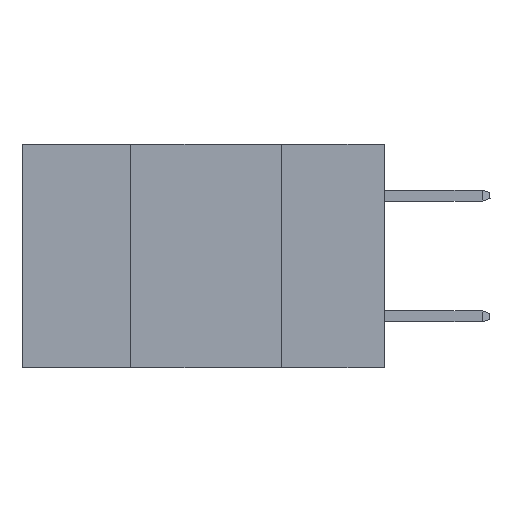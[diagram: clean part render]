
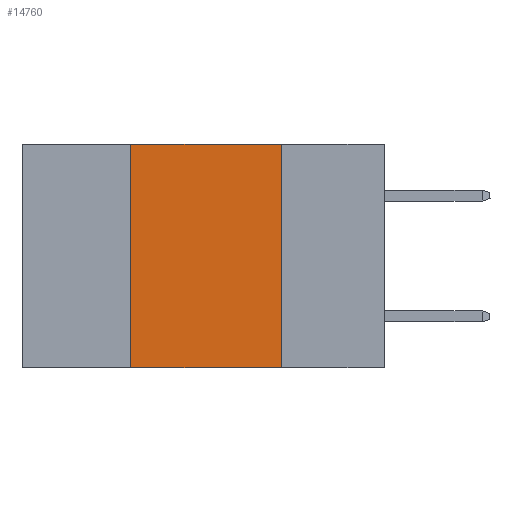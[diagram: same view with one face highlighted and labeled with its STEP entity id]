
A CAD part, left-side view. The second image highlights one B-rep face of the part: STEP entity #14760.
In plain terms, the highlighted planar face has unit normal (-1, 0, 0).
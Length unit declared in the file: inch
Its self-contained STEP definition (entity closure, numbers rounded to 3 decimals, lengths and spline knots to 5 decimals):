
#54 = LINE ( 'NONE', #14823, #1248 ) ;
#1071 = ORIENTED_EDGE ( 'NONE', *, *, #12630, .T. ) ;
#1248 = VECTOR ( 'NONE', #8306, 39.37008 ) ;
#1367 = VERTEX_POINT ( 'NONE', #11311 ) ;
#1566 = ORIENTED_EDGE ( 'NONE', *, *, #7114, .F. ) ;
#1580 = VERTEX_POINT ( 'NONE', #2949 ) ;
#1901 = CARTESIAN_POINT ( 'NONE',  ( 0., 0.42, -0.37 ) ) ;
#2280 = DIRECTION ( 'NONE',  ( 0., 0., 1. ) ) ;
#2737 = EDGE_LOOP ( 'NONE', ( #1566, #14955, #4477, #1071 ) ) ;
#2758 = CARTESIAN_POINT ( 'NONE',  ( 0., 0.17, -0.37 ) ) ;
#2822 = EDGE_CURVE ( 'NONE', #1367, #1580, #5728, .T. ) ;
#2896 = DIRECTION ( 'NONE',  ( 0., 0., -1. ) ) ;
#2917 = DIRECTION ( 'NONE',  ( 0., -1., 0. ) ) ;
#2949 = CARTESIAN_POINT ( 'NONE',  ( 0., 0.17, 0. ) ) ;
#2952 = CARTESIAN_POINT ( 'NONE',  ( 0., 0.6, 0. ) ) ;
#3183 = EDGE_CURVE ( 'NONE', #7134, #1367, #15098, .T. ) ;
#3380 = VECTOR ( 'NONE', #2280, 39.37008 ) ;
#3754 = CARTESIAN_POINT ( 'NONE',  ( 0., 0.6, 0. ) ) ;
#4282 = VECTOR ( 'NONE', #12728, 39.37008 ) ;
#4477 = ORIENTED_EDGE ( 'NONE', *, *, #3183, .F. ) ;
#5728 = LINE ( 'NONE', #3754, #4282 ) ;
#6722 = DIRECTION ( 'NONE',  ( 1., 0., 0. ) ) ;
#7114 = EDGE_CURVE ( 'NONE', #1580, #9350, #54, .T. ) ;
#7134 = VERTEX_POINT ( 'NONE', #1901 ) ;
#7384 = CARTESIAN_POINT ( 'NONE',  ( 0., 0.42, 0. ) ) ;
#8306 = DIRECTION ( 'NONE',  ( 0., 0., -1. ) ) ;
#9350 = VERTEX_POINT ( 'NONE', #2758 ) ;
#9428 = CARTESIAN_POINT ( 'NONE',  ( 0., 0.6, -0.37 ) ) ;
#11311 = CARTESIAN_POINT ( 'NONE',  ( 0., 0.42, 0. ) ) ;
#12630 = EDGE_CURVE ( 'NONE', #7134, #9350, #13034, .T. ) ;
#12728 = DIRECTION ( 'NONE',  ( 0., -1., 0. ) ) ;
#13034 = LINE ( 'NONE', #9428, #14447 ) ;
#13369 = FACE_OUTER_BOUND ( 'NONE', #2737, .T. ) ;
#14447 = VECTOR ( 'NONE', #2917, 39.37008 ) ;
#14760 = ADVANCED_FACE ( 'NONE', ( #13369 ), #15823, .F. ) ;
#14823 = CARTESIAN_POINT ( 'NONE',  ( 0., 0.17, 0. ) ) ;
#14955 = ORIENTED_EDGE ( 'NONE', *, *, #2822, .F. ) ;
#15098 = LINE ( 'NONE', #7384, #3380 ) ;
#15443 = AXIS2_PLACEMENT_3D ( 'NONE', #2952, #6722, #2896 ) ;
#15823 = PLANE ( 'NONE',  #15443 ) ;
